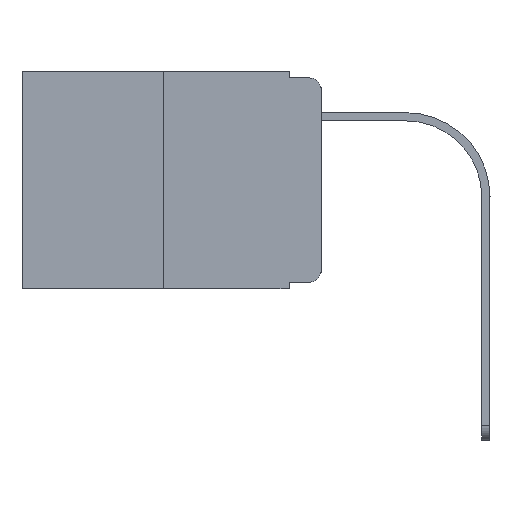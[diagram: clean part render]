
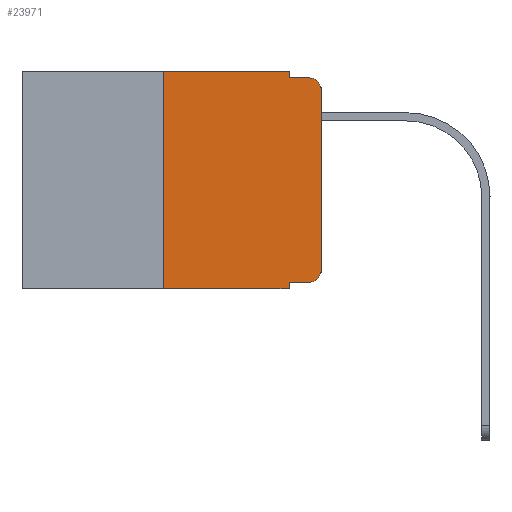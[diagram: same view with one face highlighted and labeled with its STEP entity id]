
A CAD part, left-side view. The second image highlights one B-rep face of the part: STEP entity #23971.
In plain terms, the highlighted planar face has unit normal (-1, 0, 0).
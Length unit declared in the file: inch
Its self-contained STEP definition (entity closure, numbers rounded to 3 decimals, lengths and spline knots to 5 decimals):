
#62 = VECTOR ( 'NONE', #15017, 39.37008 ) ;
#241 = DIRECTION ( 'NONE',  ( 0., 0., -1. ) ) ;
#799 = DIRECTION ( 'NONE',  ( 0., -1., 0. ) ) ;
#1288 = EDGE_CURVE ( 'NONE', #12083, #4492, #14044, .T. ) ;
#1493 = FACE_OUTER_BOUND ( 'NONE', #2431, .T. ) ;
#1594 = DIRECTION ( 'NONE',  ( 0., 0., -1. ) ) ;
#1664 = VERTEX_POINT ( 'NONE', #17900 ) ;
#1921 = ORIENTED_EDGE ( 'NONE', *, *, #1288, .T. ) ;
#1955 = VERTEX_POINT ( 'NONE', #24642 ) ;
#2031 = AXIS2_PLACEMENT_3D ( 'NONE', #11294, #5576, #1594 ) ;
#2173 = ORIENTED_EDGE ( 'NONE', *, *, #22298, .T. ) ;
#2431 = EDGE_LOOP ( 'NONE', ( #9893, #2173, #12925, #24287, #15350, #21529, #6400, #14899, #1921, #4064 ) ) ;
#2807 = CARTESIAN_POINT ( 'NONE',  ( 0., 0.02, -0.333 ) ) ;
#3080 = DIRECTION ( 'NONE',  ( 0., 0., -1. ) ) ;
#3172 = LINE ( 'NONE', #11316, #62 ) ;
#3413 = AXIS2_PLACEMENT_3D ( 'NONE', #16960, #5127, #3080 ) ;
#3434 = CIRCLE ( 'NONE', #3413, 0.02 ) ;
#3505 = DIRECTION ( 'NONE',  ( 0., 0., -1. ) ) ;
#4064 = ORIENTED_EDGE ( 'NONE', *, *, #5671, .T. ) ;
#4240 = DIRECTION ( 'NONE',  ( 0., -1., 0. ) ) ;
#4492 = VERTEX_POINT ( 'NONE', #2807 ) ;
#4603 = CARTESIAN_POINT ( 'NONE',  ( 0., 0.051, -0.333 ) ) ;
#4972 = VECTOR ( 'NONE', #9468, 39.37008 ) ;
#5102 = LINE ( 'NONE', #8789, #20047 ) ;
#5127 = DIRECTION ( 'NONE',  ( -1., 0., 0. ) ) ;
#5576 = DIRECTION ( 'NONE',  ( 1., 0., 0. ) ) ;
#5671 = EDGE_CURVE ( 'NONE', #4492, #17294, #3434, .T. ) ;
#6083 = DIRECTION ( 'NONE',  ( -1., 0., 0. ) ) ;
#6283 = LINE ( 'NONE', #10227, #10738 ) ;
#6400 = ORIENTED_EDGE ( 'NONE', *, *, #24210, .T. ) ;
#6919 = CARTESIAN_POINT ( 'NONE',  ( 0., 0.051, 0. ) ) ;
#7426 = CARTESIAN_POINT ( 'NONE',  ( 0., 0.051, -0.01 ) ) ;
#8234 = VECTOR ( 'NONE', #23944, 39.37008 ) ;
#8789 = CARTESIAN_POINT ( 'NONE',  ( 0., 0.473, 0. ) ) ;
#8905 = VERTEX_POINT ( 'NONE', #21228 ) ;
#9468 = DIRECTION ( 'NONE',  ( 0., -1., 0. ) ) ;
#9893 = ORIENTED_EDGE ( 'NONE', *, *, #16685, .T. ) ;
#10227 = CARTESIAN_POINT ( 'NONE',  ( 0., 0.25, 0. ) ) ;
#10239 = EDGE_CURVE ( 'NONE', #19730, #1664, #24814, .T. ) ;
#10738 = VECTOR ( 'NONE', #23336, 39.37008 ) ;
#11294 = CARTESIAN_POINT ( 'NONE',  ( 0., 0.473, 0. ) ) ;
#11316 = CARTESIAN_POINT ( 'NONE',  ( 0., 0.051, 0. ) ) ;
#12083 = VERTEX_POINT ( 'NONE', #15792 ) ;
#12687 = EDGE_CURVE ( 'NONE', #12083, #14104, #24324, .T. ) ;
#12713 = DIRECTION ( 'NONE',  ( 0., -1., 0. ) ) ;
#12925 = ORIENTED_EDGE ( 'NONE', *, *, #10239, .F. ) ;
#14044 = LINE ( 'NONE', #4603, #17579 ) ;
#14104 = VERTEX_POINT ( 'NONE', #17506 ) ;
#14680 = EDGE_CURVE ( 'NONE', #23004, #19730, #3172, .T. ) ;
#14899 = ORIENTED_EDGE ( 'NONE', *, *, #12687, .F. ) ;
#15017 = DIRECTION ( 'NONE',  ( 0., 0., -1. ) ) ;
#15283 = CARTESIAN_POINT ( 'NONE',  ( 0., 0., -0.03 ) ) ;
#15350 = ORIENTED_EDGE ( 'NONE', *, *, #17119, .F. ) ;
#15385 = CARTESIAN_POINT ( 'NONE',  ( 0., 0.02, -0.03 ) ) ;
#15792 = CARTESIAN_POINT ( 'NONE',  ( 0., 0.051, -0.333 ) ) ;
#16106 = LINE ( 'NONE', #18129, #8234 ) ;
#16240 = VECTOR ( 'NONE', #799, 39.37008 ) ;
#16685 = EDGE_CURVE ( 'NONE', #17294, #17267, #16106, .T. ) ;
#16875 = VECTOR ( 'NONE', #3505, 39.37008 ) ;
#16960 = CARTESIAN_POINT ( 'NONE',  ( 0., 0.02, -0.313 ) ) ;
#17119 = EDGE_CURVE ( 'NONE', #8905, #23004, #5102, .T. ) ;
#17267 = VERTEX_POINT ( 'NONE', #15283 ) ;
#17294 = VERTEX_POINT ( 'NONE', #21094 ) ;
#17506 = CARTESIAN_POINT ( 'NONE',  ( 0., 0.051, -0.343 ) ) ;
#17579 = VECTOR ( 'NONE', #4240, 39.37008 ) ;
#17900 = CARTESIAN_POINT ( 'NONE',  ( 0., 0.02, -0.01 ) ) ;
#18115 = AXIS2_PLACEMENT_3D ( 'NONE', #15385, #6083, #241 ) ;
#18129 = CARTESIAN_POINT ( 'NONE',  ( 0., 0., 0. ) ) ;
#18356 = LINE ( 'NONE', #19901, #16240 ) ;
#19699 = EDGE_CURVE ( 'NONE', #1955, #8905, #6283, .T. ) ;
#19730 = VERTEX_POINT ( 'NONE', #23190 ) ;
#19901 = CARTESIAN_POINT ( 'NONE',  ( 0., 0.473, -0.343 ) ) ;
#20047 = VECTOR ( 'NONE', #12713, 39.37008 ) ;
#20671 = PLANE ( 'NONE',  #2031 ) ;
#21094 = CARTESIAN_POINT ( 'NONE',  ( 0., 0., -0.313 ) ) ;
#21228 = CARTESIAN_POINT ( 'NONE',  ( 0., 0.25, 0. ) ) ;
#21529 = ORIENTED_EDGE ( 'NONE', *, *, #19699, .F. ) ;
#21810 = CARTESIAN_POINT ( 'NONE',  ( 0., 0.051, 0. ) ) ;
#22298 = EDGE_CURVE ( 'NONE', #17267, #1664, #22973, .T. ) ;
#22973 = CIRCLE ( 'NONE', #18115, 0.02 ) ;
#23004 = VERTEX_POINT ( 'NONE', #21810 ) ;
#23190 = CARTESIAN_POINT ( 'NONE',  ( 0., 0.051, -0.01 ) ) ;
#23336 = DIRECTION ( 'NONE',  ( 0., 0., 1. ) ) ;
#23944 = DIRECTION ( 'NONE',  ( 0., 0., 1. ) ) ;
#23971 = ADVANCED_FACE ( 'NONE', ( #1493 ), #20671, .F. ) ;
#24210 = EDGE_CURVE ( 'NONE', #1955, #14104, #18356, .T. ) ;
#24287 = ORIENTED_EDGE ( 'NONE', *, *, #14680, .F. ) ;
#24324 = LINE ( 'NONE', #6919, #16875 ) ;
#24642 = CARTESIAN_POINT ( 'NONE',  ( 0., 0.25, -0.343 ) ) ;
#24814 = LINE ( 'NONE', #7426, #4972 ) ;
